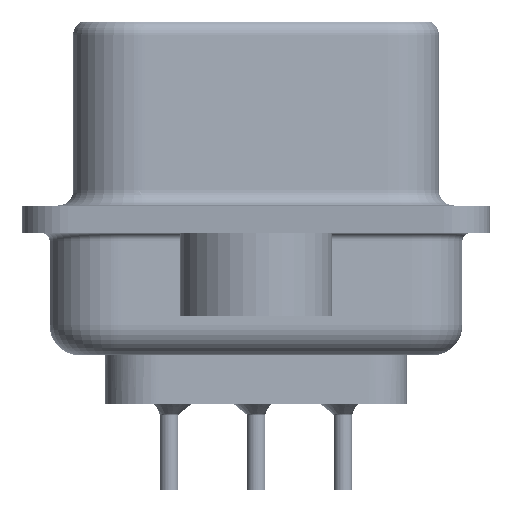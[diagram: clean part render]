
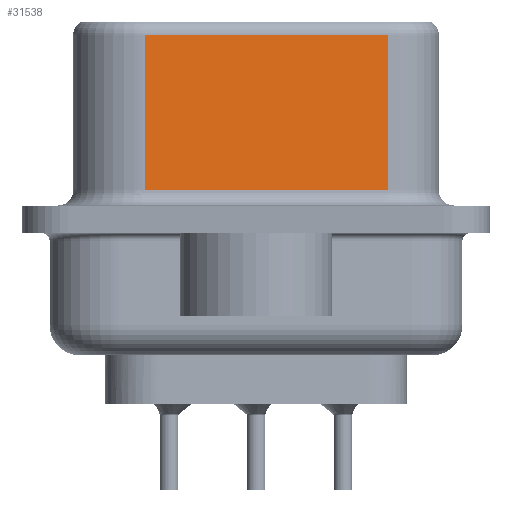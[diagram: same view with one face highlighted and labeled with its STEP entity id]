
A CAD part, left-side view. The second image highlights one B-rep face of the part: STEP entity #31538.
In plain terms, the highlighted planar face has unit normal (-0.985, -0.174, 0).
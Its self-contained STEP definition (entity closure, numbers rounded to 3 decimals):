
#1392 = CARTESIAN_POINT ( 'NONE',  ( 5.132, -4.322, 6.52 ) ) ;
#1568 = ORIENTED_EDGE ( 'NONE', *, *, #11531, .T. ) ;
#2233 = CARTESIAN_POINT ( 'NONE',  ( 5.132, -4.322, 0.95 ) ) ;
#2418 = CARTESIAN_POINT ( 'NONE',  ( 3.73, 3.628, 6.02 ) ) ;
#4185 = PLANE ( 'NONE',  #19572 ) ;
#4657 = VECTOR ( 'NONE', #5025, 1000. ) ;
#5025 = DIRECTION ( 'NONE',  ( 0.174, -0.985, 0. ) ) ;
#5074 = VERTEX_POINT ( 'NONE', #14782 ) ;
#5293 = EDGE_CURVE ( 'NONE', #32527, #5074, #28982, .T. ) ;
#6964 = DIRECTION ( 'NONE',  ( 0.985, 0.174, 0. ) ) ;
#7908 = VECTOR ( 'NONE', #27463, 1000. ) ;
#8580 = DIRECTION ( 'NONE',  ( -0.174, 0.985, 0. ) ) ;
#8746 = ORIENTED_EDGE ( 'NONE', *, *, #19506, .T. ) ;
#8947 = VECTOR ( 'NONE', #25768, 1000. ) ;
#10836 = VECTOR ( 'NONE', #8580, 1000. ) ;
#10995 = CARTESIAN_POINT ( 'NONE',  ( 5.132, -4.322, 6.52 ) ) ;
#11531 = EDGE_CURVE ( 'NONE', #35184, #5074, #11990, .T. ) ;
#11714 = LINE ( 'NONE', #30411, #10836 ) ;
#11990 = LINE ( 'NONE', #2233, #4657 ) ;
#12764 = CARTESIAN_POINT ( 'NONE',  ( 5.132, -4.322, 6.02 ) ) ;
#14687 = ORIENTED_EDGE ( 'NONE', *, *, #5293, .F. ) ;
#14782 = CARTESIAN_POINT ( 'NONE',  ( 5.132, -4.322, 0.95 ) ) ;
#16561 = EDGE_CURVE ( 'NONE', #32527, #30553, #11714, .T. ) ;
#17127 = LINE ( 'NONE', #20237, #8947 ) ;
#18275 = ORIENTED_EDGE ( 'NONE', *, *, #16561, .T. ) ;
#18435 = FACE_OUTER_BOUND ( 'NONE', #18755, .T. ) ;
#18755 = EDGE_LOOP ( 'NONE', ( #14687, #18275, #8746, #1568 ) ) ;
#19506 = EDGE_CURVE ( 'NONE', #30553, #35184, #17127, .T. ) ;
#19572 = AXIS2_PLACEMENT_3D ( 'NONE', #1392, #6964, #26205 ) ;
#20237 = CARTESIAN_POINT ( 'NONE',  ( 3.73, 3.628, 6.52 ) ) ;
#21168 = CARTESIAN_POINT ( 'NONE',  ( 3.73, 3.628, 0.95 ) ) ;
#25768 = DIRECTION ( 'NONE',  ( 0., 0., -1. ) ) ;
#26205 = DIRECTION ( 'NONE',  ( -0.174, 0.985, 0. ) ) ;
#27463 = DIRECTION ( 'NONE',  ( 0., 0., -1. ) ) ;
#28982 = LINE ( 'NONE', #10995, #7908 ) ;
#30411 = CARTESIAN_POINT ( 'NONE',  ( 5.132, -4.322, 6.02 ) ) ;
#30553 = VERTEX_POINT ( 'NONE', #2418 ) ;
#31538 = ADVANCED_FACE ( 'NONE', ( #18435 ), #4185, .F. ) ;
#32527 = VERTEX_POINT ( 'NONE', #12764 ) ;
#35184 = VERTEX_POINT ( 'NONE', #21168 ) ;
